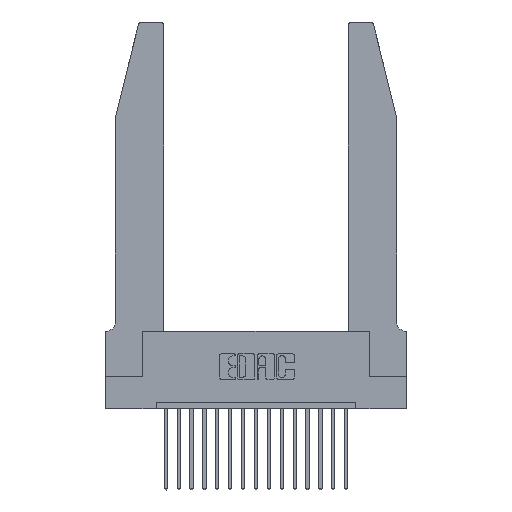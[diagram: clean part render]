
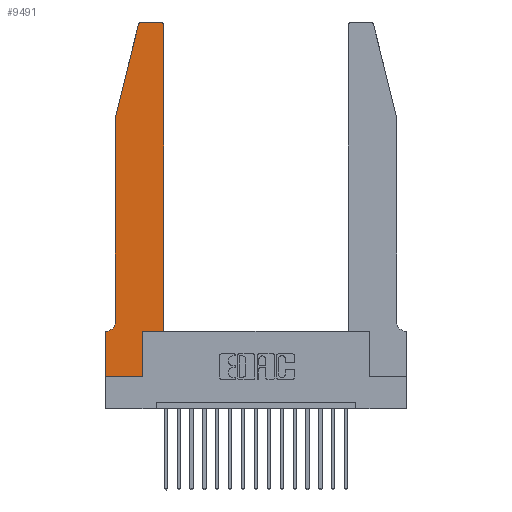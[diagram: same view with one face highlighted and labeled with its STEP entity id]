
A CAD part, top view. The second image highlights one B-rep face of the part: STEP entity #9491.
In plain terms, the highlighted planar face has unit normal (0, 0, 1).
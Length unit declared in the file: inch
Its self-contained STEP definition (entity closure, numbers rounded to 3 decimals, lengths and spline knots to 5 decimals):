
#172 = DIRECTION ( 'NONE',  ( -0.239, -0.971, 0. ) ) ;
#453 = DIRECTION ( 'NONE',  ( -1., 0., 0. ) ) ;
#478 = CARTESIAN_POINT ( 'NONE',  ( 0.2605, 2.75, 0.37 ) ) ;
#646 = CARTESIAN_POINT ( 'NONE',  ( 0.2865, 0.35, 0.37 ) ) ;
#656 = VECTOR ( 'NONE', #11437, 39.37008 ) ;
#894 = CARTESIAN_POINT ( 'NONE',  ( 0.284, 2.72, 0.37 ) ) ;
#921 = AXIS2_PLACEMENT_3D ( 'NONE', #6671, #3566, #453 ) ;
#962 = DIRECTION ( 'NONE',  ( 1., 0., 0. ) ) ;
#970 = LINE ( 'NONE', #19723, #3828 ) ;
#1433 = VECTOR ( 'NONE', #9144, 39.37008 ) ;
#1457 = EDGE_CURVE ( 'NONE', #10305, #5764, #15040, .T. ) ;
#1577 = CARTESIAN_POINT ( 'NONE',  ( 0.4505, 0.35, 0.37 ) ) ;
#1698 = VERTEX_POINT ( 'NONE', #5119 ) ;
#2296 = CARTESIAN_POINT ( 'NONE',  ( 0.4505, 0.35, 0.37 ) ) ;
#2414 = DIRECTION ( 'NONE',  ( 0., 0., 1. ) ) ;
#2530 = CARTESIAN_POINT ( 'NONE',  ( 0.2865, 0., 0.37 ) ) ;
#2543 = EDGE_CURVE ( 'NONE', #5764, #11905, #12267, .T. ) ;
#2582 = VERTEX_POINT ( 'NONE', #11107 ) ;
#2941 = ORIENTED_EDGE ( 'NONE', *, *, #17798, .T. ) ;
#3090 = VERTEX_POINT ( 'NONE', #5725 ) ;
#3098 = CARTESIAN_POINT ( 'NONE',  ( 0.0755, 2., 0.37 ) ) ;
#3566 = DIRECTION ( 'NONE',  ( 0., 0., -1. ) ) ;
#3828 = VECTOR ( 'NONE', #10476, 39.37008 ) ;
#3857 = CARTESIAN_POINT ( 'NONE',  ( 0.0755, 2., 0.37 ) ) ;
#3922 = ORIENTED_EDGE ( 'NONE', *, *, #1457, .T. ) ;
#4252 = LINE ( 'NONE', #3098, #16873 ) ;
#4287 = VERTEX_POINT ( 'NONE', #6537 ) ;
#4478 = AXIS2_PLACEMENT_3D ( 'NONE', #5321, #12938, #962 ) ;
#4663 = LINE ( 'NONE', #3857, #656 ) ;
#5119 = CARTESIAN_POINT ( 'NONE',  ( 0., 0.35, 0.37 ) ) ;
#5321 = CARTESIAN_POINT ( 'NONE',  ( 0., 0.35, 0.37 ) ) ;
#5725 = CARTESIAN_POINT ( 'NONE',  ( 0.4205, 2.75, 0.37 ) ) ;
#5764 = VERTEX_POINT ( 'NONE', #646 ) ;
#5960 = LINE ( 'NONE', #478, #17156 ) ;
#6260 = CARTESIAN_POINT ( 'NONE',  ( 0.2865, 0.35, 0.37 ) ) ;
#6537 = CARTESIAN_POINT ( 'NONE',  ( 0.0755, 0.42, 0.37 ) ) ;
#6671 = CARTESIAN_POINT ( 'NONE',  ( 0.0055, 0.42, 0.37 ) ) ;
#6707 = CARTESIAN_POINT ( 'NONE',  ( 0.4205, 2.72, 0.37 ) ) ;
#6757 = CARTESIAN_POINT ( 'NONE',  ( 0.0755, 2., 0.37 ) ) ;
#6817 = EDGE_CURVE ( 'NONE', #8980, #3090, #10420, .T. ) ;
#7078 = VERTEX_POINT ( 'NONE', #17882 ) ;
#7178 = VECTOR ( 'NONE', #9339, 39.37008 ) ;
#8035 = LINE ( 'NONE', #9197, #11801 ) ;
#8081 = VERTEX_POINT ( 'NONE', #6757 ) ;
#8111 = DIRECTION ( 'NONE',  ( 0., 0., 1. ) ) ;
#8363 = FACE_OUTER_BOUND ( 'NONE', #8477, .T. ) ;
#8364 = ORIENTED_EDGE ( 'NONE', *, *, #13871, .T. ) ;
#8477 = EDGE_LOOP ( 'NONE', ( #11926, #12182, #11550, #8364, #12773, #10408, #11591, #2941, #3922, #18412, #17126, #9662 ) ) ;
#8908 = EDGE_CURVE ( 'NONE', #3090, #11764, #5960, .T. ) ;
#8954 = VECTOR ( 'NONE', #15711, 39.37008 ) ;
#8980 = VERTEX_POINT ( 'NONE', #14592 ) ;
#9144 = DIRECTION ( 'NONE',  ( 0., 1., 0. ) ) ;
#9197 = CARTESIAN_POINT ( 'NONE',  ( 0., 0., 0.37 ) ) ;
#9339 = DIRECTION ( 'NONE',  ( 0., 1., 0. ) ) ;
#9491 = ADVANCED_FACE ( 'NONE', ( #8363 ), #11584, .T. ) ;
#9531 = EDGE_CURVE ( 'NONE', #11764, #7078, #19116, .T. ) ;
#9662 = ORIENTED_EDGE ( 'NONE', *, *, #6817, .T. ) ;
#10305 = VERTEX_POINT ( 'NONE', #2530 ) ;
#10408 = ORIENTED_EDGE ( 'NONE', *, *, #11799, .T. ) ;
#10420 = CIRCLE ( 'NONE', #14961, 0.03 ) ;
#10476 = DIRECTION ( 'NONE',  ( -1., 0., 0. ) ) ;
#11094 = LINE ( 'NONE', #1577, #1433 ) ;
#11107 = CARTESIAN_POINT ( 'NONE',  ( 0., 0., 0.37 ) ) ;
#11303 = DIRECTION ( 'NONE',  ( 1., 0., 0. ) ) ;
#11320 = CARTESIAN_POINT ( 'NONE',  ( 0., 0., 0.37 ) ) ;
#11437 = DIRECTION ( 'NONE',  ( 0., -1., 0. ) ) ;
#11550 = ORIENTED_EDGE ( 'NONE', *, *, #17460, .T. ) ;
#11584 = PLANE ( 'NONE',  #4478 ) ;
#11591 = ORIENTED_EDGE ( 'NONE', *, *, #18257, .T. ) ;
#11764 = VERTEX_POINT ( 'NONE', #11958 ) ;
#11799 = EDGE_CURVE ( 'NONE', #14924, #1698, #970, .T. ) ;
#11801 = VECTOR ( 'NONE', #16892, 39.37008 ) ;
#11905 = VERTEX_POINT ( 'NONE', #2296 ) ;
#11926 = ORIENTED_EDGE ( 'NONE', *, *, #8908, .T. ) ;
#11958 = CARTESIAN_POINT ( 'NONE',  ( 0.284, 2.75, 0.37 ) ) ;
#12050 = LINE ( 'NONE', #11320, #8954 ) ;
#12182 = ORIENTED_EDGE ( 'NONE', *, *, #9531, .T. ) ;
#12267 = LINE ( 'NONE', #14167, #15174 ) ;
#12773 = ORIENTED_EDGE ( 'NONE', *, *, #19614, .T. ) ;
#12938 = DIRECTION ( 'NONE',  ( 0., 0., 1. ) ) ;
#13871 = EDGE_CURVE ( 'NONE', #8081, #4287, #4663, .T. ) ;
#14167 = CARTESIAN_POINT ( 'NONE',  ( 0.4505, 0.35, 0.37 ) ) ;
#14592 = CARTESIAN_POINT ( 'NONE',  ( 0.4505, 2.72, 0.37 ) ) ;
#14874 = CIRCLE ( 'NONE', #921, 0.07 ) ;
#14924 = VERTEX_POINT ( 'NONE', #18497 ) ;
#14961 = AXIS2_PLACEMENT_3D ( 'NONE', #6707, #8111, #11303 ) ;
#15040 = LINE ( 'NONE', #6260, #7178 ) ;
#15174 = VECTOR ( 'NONE', #18593, 39.37008 ) ;
#15711 = DIRECTION ( 'NONE',  ( 1., 0., 0. ) ) ;
#16170 = DIRECTION ( 'NONE',  ( 1., 0., 0. ) ) ;
#16873 = VECTOR ( 'NONE', #172, 39.37008 ) ;
#16892 = DIRECTION ( 'NONE',  ( 0., -1., 0. ) ) ;
#17126 = ORIENTED_EDGE ( 'NONE', *, *, #17610, .T. ) ;
#17156 = VECTOR ( 'NONE', #19146, 39.37008 ) ;
#17460 = EDGE_CURVE ( 'NONE', #7078, #8081, #4252, .T. ) ;
#17610 = EDGE_CURVE ( 'NONE', #11905, #8980, #11094, .T. ) ;
#17741 = AXIS2_PLACEMENT_3D ( 'NONE', #894, #2414, #16170 ) ;
#17798 = EDGE_CURVE ( 'NONE', #2582, #10305, #12050, .T. ) ;
#17882 = CARTESIAN_POINT ( 'NONE',  ( 0.25487, 2.72718, 0.37 ) ) ;
#18257 = EDGE_CURVE ( 'NONE', #1698, #2582, #8035, .T. ) ;
#18412 = ORIENTED_EDGE ( 'NONE', *, *, #2543, .T. ) ;
#18497 = CARTESIAN_POINT ( 'NONE',  ( 0.0055, 0.35, 0.37 ) ) ;
#18593 = DIRECTION ( 'NONE',  ( 1., 0., 0. ) ) ;
#19116 = CIRCLE ( 'NONE', #17741, 0.03 ) ;
#19146 = DIRECTION ( 'NONE',  ( -1., 0., 0. ) ) ;
#19614 = EDGE_CURVE ( 'NONE', #4287, #14924, #14874, .T. ) ;
#19723 = CARTESIAN_POINT ( 'NONE',  ( 0.0755, 0.35, 0.37 ) ) ;
